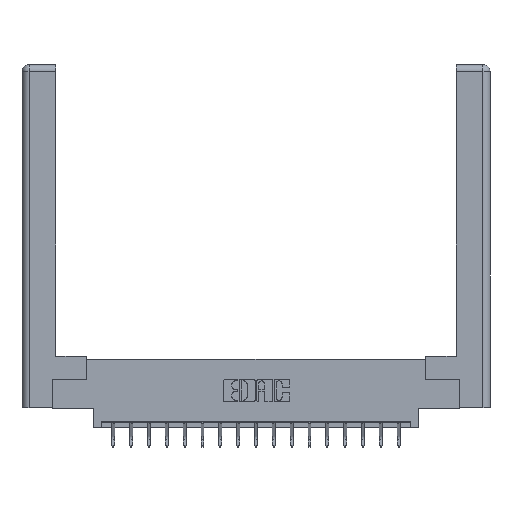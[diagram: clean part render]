
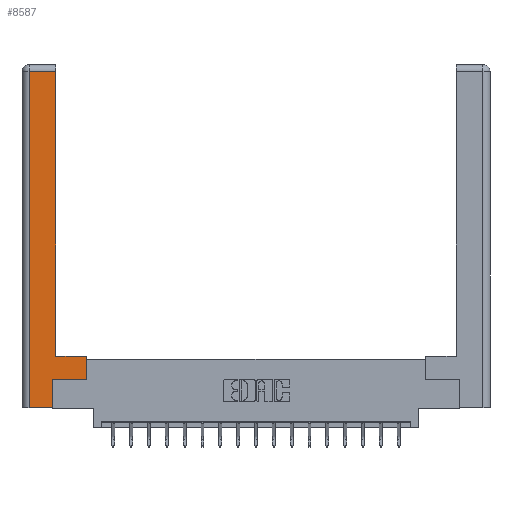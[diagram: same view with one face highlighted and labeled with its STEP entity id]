
A CAD part, top view. The second image highlights one B-rep face of the part: STEP entity #8587.
In plain terms, the highlighted planar face has unit normal (0, 0, 1).
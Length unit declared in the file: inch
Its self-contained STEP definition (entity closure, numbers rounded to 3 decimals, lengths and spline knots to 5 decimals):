
#592 = ORIENTED_EDGE ( 'NONE', *, *, #4509, .T. ) ;
#829 = VECTOR ( 'NONE', #9697, 39.37008 ) ;
#841 = ORIENTED_EDGE ( 'NONE', *, *, #2197, .T. ) ;
#1274 = VERTEX_POINT ( 'NONE', #8542 ) ;
#1764 = CARTESIAN_POINT ( 'NONE',  ( 0.565, 0.245, 0. ) ) ;
#1808 = EDGE_CURVE ( 'NONE', #2536, #19420, #14472, .T. ) ;
#1837 = AXIS2_PLACEMENT_3D ( 'NONE', #15944, #5646, #17592 ) ;
#2197 = EDGE_CURVE ( 'NONE', #19420, #18290, #5085, .T. ) ;
#2238 = VECTOR ( 'NONE', #11636, 39.37008 ) ;
#2501 = ORIENTED_EDGE ( 'NONE', *, *, #6098, .T. ) ;
#2536 = VERTEX_POINT ( 'NONE', #14582 ) ;
#2700 = EDGE_CURVE ( 'NONE', #18145, #1274, #19085, .T. ) ;
#2886 = EDGE_CURVE ( 'NONE', #18290, #10270, #16735, .T. ) ;
#3722 = EDGE_LOOP ( 'NONE', ( #592, #9562, #8069, #9399, #841, #8089, #2501, #4414 ) ) ;
#4275 = CARTESIAN_POINT ( 'NONE',  ( 0.565, 0.45, 0. ) ) ;
#4414 = ORIENTED_EDGE ( 'NONE', *, *, #2700, .T. ) ;
#4509 = EDGE_CURVE ( 'NONE', #1274, #9970, #15253, .T. ) ;
#4755 = DIRECTION ( 'NONE',  ( 0., -1., 0. ) ) ;
#5085 = LINE ( 'NONE', #12239, #8606 ) ;
#5646 = DIRECTION ( 'NONE',  ( 0., 0., -1. ) ) ;
#5759 = LINE ( 'NONE', #13185, #2238 ) ;
#6098 = EDGE_CURVE ( 'NONE', #10270, #18145, #18253, .T. ) ;
#6373 = DIRECTION ( 'NONE',  ( 0., 1., 0. ) ) ;
#6385 = DIRECTION ( 'NONE',  ( 1., 0., 0. ) ) ;
#6853 = VECTOR ( 'NONE', #7892, 39.37008 ) ;
#6947 = VECTOR ( 'NONE', #8475, 39.37008 ) ;
#7168 = VERTEX_POINT ( 'NONE', #8773 ) ;
#7892 = DIRECTION ( 'NONE',  ( 0., 1., 0. ) ) ;
#8069 = ORIENTED_EDGE ( 'NONE', *, *, #17273, .T. ) ;
#8089 = ORIENTED_EDGE ( 'NONE', *, *, #2886, .T. ) ;
#8475 = DIRECTION ( 'NONE',  ( -1., 0., 0. ) ) ;
#8542 = CARTESIAN_POINT ( 'NONE',  ( 0.295, 0.45, 0. ) ) ;
#8587 = ADVANCED_FACE ( 'NONE', ( #18474 ), #13948, .F. ) ;
#8606 = VECTOR ( 'NONE', #6373, 39.37008 ) ;
#8773 = CARTESIAN_POINT ( 'NONE',  ( 0.0615, 2.94, 0. ) ) ;
#9399 = ORIENTED_EDGE ( 'NONE', *, *, #1808, .T. ) ;
#9562 = ORIENTED_EDGE ( 'NONE', *, *, #15268, .T. ) ;
#9697 = DIRECTION ( 'NONE',  ( 1., 0., 0. ) ) ;
#9970 = VERTEX_POINT ( 'NONE', #13055 ) ;
#10270 = VERTEX_POINT ( 'NONE', #13781 ) ;
#11331 = CARTESIAN_POINT ( 'NONE',  ( 0.295, 0.45, 0. ) ) ;
#11636 = DIRECTION ( 'NONE',  ( -1., 0., 0. ) ) ;
#12239 = CARTESIAN_POINT ( 'NONE',  ( 0.265, 0.245, 0. ) ) ;
#12832 = DIRECTION ( 'NONE',  ( 0., 1., 0. ) ) ;
#13055 = CARTESIAN_POINT ( 'NONE',  ( 0.295, 2.94, 0. ) ) ;
#13185 = CARTESIAN_POINT ( 'NONE',  ( 0.0615, 2.94, 0. ) ) ;
#13740 = CARTESIAN_POINT ( 'NONE',  ( 0.265, 0.245, 0. ) ) ;
#13781 = CARTESIAN_POINT ( 'NONE',  ( 0.565, 0.245, 0. ) ) ;
#13948 = PLANE ( 'NONE',  #1837 ) ;
#14472 = LINE ( 'NONE', #18611, #829 ) ;
#14582 = CARTESIAN_POINT ( 'NONE',  ( 0.0615, 0., 0. ) ) ;
#15253 = LINE ( 'NONE', #18353, #6853 ) ;
#15268 = EDGE_CURVE ( 'NONE', #9970, #7168, #5759, .T. ) ;
#15714 = CARTESIAN_POINT ( 'NONE',  ( 0.565, 0.45, 0. ) ) ;
#15944 = CARTESIAN_POINT ( 'NONE',  ( 0., 0., 0. ) ) ;
#16658 = CARTESIAN_POINT ( 'NONE',  ( 0.265, 0., 0. ) ) ;
#16735 = LINE ( 'NONE', #1764, #17428 ) ;
#17273 = EDGE_CURVE ( 'NONE', #7168, #2536, #19005, .T. ) ;
#17428 = VECTOR ( 'NONE', #6385, 39.37008 ) ;
#17592 = DIRECTION ( 'NONE',  ( -1., 0., 0. ) ) ;
#18145 = VERTEX_POINT ( 'NONE', #4275 ) ;
#18166 = CARTESIAN_POINT ( 'NONE',  ( 0.0615, 0., 0. ) ) ;
#18253 = LINE ( 'NONE', #15714, #18709 ) ;
#18290 = VERTEX_POINT ( 'NONE', #13740 ) ;
#18353 = CARTESIAN_POINT ( 'NONE',  ( 0.295, 3., 0. ) ) ;
#18474 = FACE_OUTER_BOUND ( 'NONE', #3722, .T. ) ;
#18611 = CARTESIAN_POINT ( 'NONE',  ( 0.265, 0., 0. ) ) ;
#18709 = VECTOR ( 'NONE', #12832, 39.37008 ) ;
#18768 = VECTOR ( 'NONE', #4755, 39.37008 ) ;
#19005 = LINE ( 'NONE', #18166, #18768 ) ;
#19085 = LINE ( 'NONE', #11331, #6947 ) ;
#19420 = VERTEX_POINT ( 'NONE', #16658 ) ;
